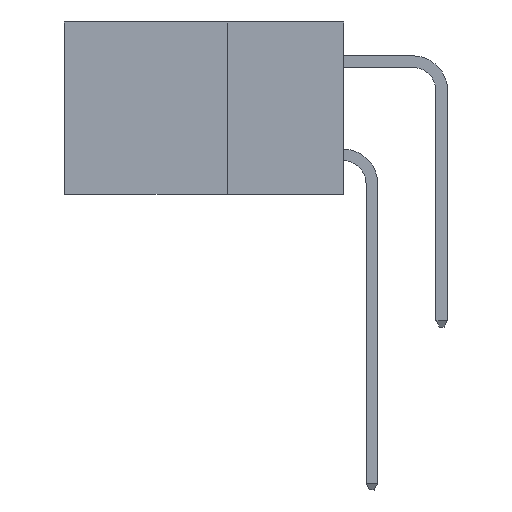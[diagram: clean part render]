
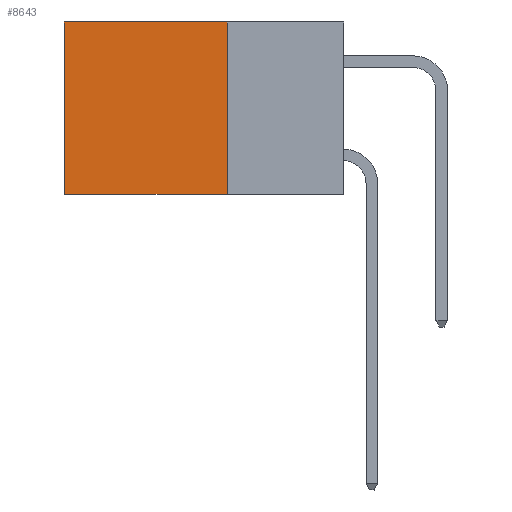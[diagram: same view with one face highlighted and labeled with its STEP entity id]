
A CAD part, left-side view. The second image highlights one B-rep face of the part: STEP entity #8643.
In plain terms, the highlighted planar face has unit normal (-1, 0, 0).
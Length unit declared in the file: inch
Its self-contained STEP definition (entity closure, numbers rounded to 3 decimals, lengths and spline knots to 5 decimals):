
#72 = CARTESIAN_POINT ( 'NONE',  ( 0.2615, 0.25, 0. ) ) ;
#78 = PLANE ( 'NONE',  #14592 ) ;
#993 = CARTESIAN_POINT ( 'NONE',  ( 0.2615, 0.25, -0.37 ) ) ;
#1315 = VECTOR ( 'NONE', #2314, 39.37008 ) ;
#1520 = CARTESIAN_POINT ( 'NONE',  ( 0.2615, 0.25, -0.37 ) ) ;
#2228 = ORIENTED_EDGE ( 'NONE', *, *, #14612, .T. ) ;
#2314 = DIRECTION ( 'NONE',  ( 0., 1., 0. ) ) ;
#2366 = CARTESIAN_POINT ( 'NONE',  ( 0.2615, 0.6, -0.37 ) ) ;
#2435 = VECTOR ( 'NONE', #9321, 39.37008 ) ;
#2742 = EDGE_CURVE ( 'NONE', #13705, #8533, #3892, .T. ) ;
#2898 = LINE ( 'NONE', #7566, #12655 ) ;
#3892 = LINE ( 'NONE', #72, #10043 ) ;
#4260 = EDGE_CURVE ( 'NONE', #4534, #10345, #8127, .T. ) ;
#4534 = VERTEX_POINT ( 'NONE', #993 ) ;
#4856 = ORIENTED_EDGE ( 'NONE', *, *, #4260, .F. ) ;
#5039 = DIRECTION ( 'NONE',  ( 1., 0., 0. ) ) ;
#6093 = LINE ( 'NONE', #2366, #2435 ) ;
#6734 = ORIENTED_EDGE ( 'NONE', *, *, #2742, .T. ) ;
#7541 = ORIENTED_EDGE ( 'NONE', *, *, #8797, .F. ) ;
#7566 = CARTESIAN_POINT ( 'NONE',  ( 0.2615, 0.25, -0.37 ) ) ;
#8127 = LINE ( 'NONE', #12792, #1315 ) ;
#8533 = VERTEX_POINT ( 'NONE', #13933 ) ;
#8643 = ADVANCED_FACE ( 'NONE', ( #14085 ), #78, .F. ) ;
#8797 = EDGE_CURVE ( 'NONE', #13705, #4534, #2898, .T. ) ;
#9321 = DIRECTION ( 'NONE',  ( 0., 0., -1. ) ) ;
#10043 = VECTOR ( 'NONE', #12849, 39.37008 ) ;
#10345 = VERTEX_POINT ( 'NONE', #14371 ) ;
#10379 = EDGE_LOOP ( 'NONE', ( #2228, #4856, #7541, #6734 ) ) ;
#12655 = VECTOR ( 'NONE', #14687, 39.37008 ) ;
#12792 = CARTESIAN_POINT ( 'NONE',  ( 0.2615, 0.25, -0.37 ) ) ;
#12849 = DIRECTION ( 'NONE',  ( 0., 1., 0. ) ) ;
#13012 = DIRECTION ( 'NONE',  ( 0., 0., -1. ) ) ;
#13705 = VERTEX_POINT ( 'NONE', #15115 ) ;
#13933 = CARTESIAN_POINT ( 'NONE',  ( 0.2615, 0.6, 0. ) ) ;
#14085 = FACE_OUTER_BOUND ( 'NONE', #10379, .T. ) ;
#14371 = CARTESIAN_POINT ( 'NONE',  ( 0.2615, 0.6, -0.37 ) ) ;
#14592 = AXIS2_PLACEMENT_3D ( 'NONE', #1520, #5039, #13012 ) ;
#14612 = EDGE_CURVE ( 'NONE', #8533, #10345, #6093, .T. ) ;
#14687 = DIRECTION ( 'NONE',  ( 0., 0., -1. ) ) ;
#15115 = CARTESIAN_POINT ( 'NONE',  ( 0.2615, 0.25, 0. ) ) ;
